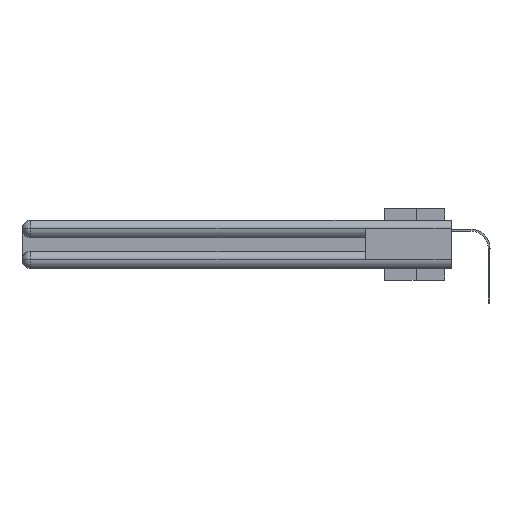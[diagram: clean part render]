
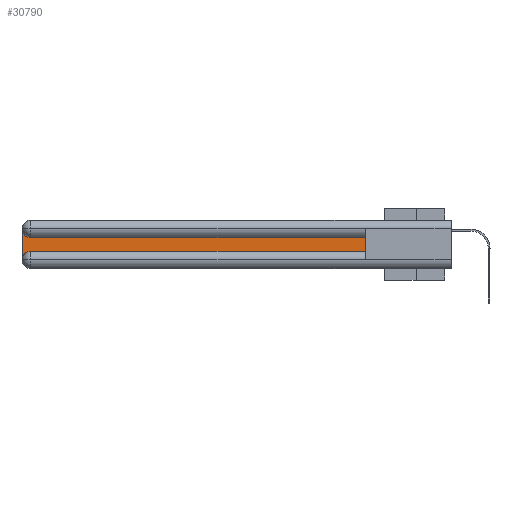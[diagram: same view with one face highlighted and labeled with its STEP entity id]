
A CAD part, left-side view. The second image highlights one B-rep face of the part: STEP entity #30790.
In plain terms, the highlighted planar face has unit normal (-1, 0, 0).
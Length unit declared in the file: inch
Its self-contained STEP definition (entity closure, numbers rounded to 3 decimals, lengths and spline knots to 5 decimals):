
#3 = EDGE_LOOP ( 'NONE', ( #7706, #17827, #25872, #24058, #19139, #547 ) ) ;
#547 = ORIENTED_EDGE ( 'NONE', *, *, #1718, .T. ) ;
#622 = DIRECTION ( 'NONE',  ( 0., 0., 1. ) ) ;
#997 = CARTESIAN_POINT ( 'NONE',  ( 0.075, 0.6, -0.1225 ) ) ;
#1361 = FACE_OUTER_BOUND ( 'NONE', #3, .T. ) ;
#1718 = EDGE_CURVE ( 'NONE', #11666, #32414, #20734, .T. ) ;
#3268 = VECTOR ( 'NONE', #26755, 39.37008 ) ;
#3394 = CARTESIAN_POINT ( 'NONE',  ( 0.075, 0.6, -0.1225 ) ) ;
#4124 = CARTESIAN_POINT ( 'NONE',  ( 0.075, 0.6, -0.2175 ) ) ;
#4169 = DIRECTION ( 'NONE',  ( 1., 0., 0. ) ) ;
#5726 = DIRECTION ( 'NONE',  ( 0., 0., -1. ) ) ;
#5893 = AXIS2_PLACEMENT_3D ( 'NONE', #29638, #4169, #29796 ) ;
#6067 = VERTEX_POINT ( 'NONE', #24082 ) ;
#6148 = VECTOR ( 'NONE', #622, 39.37008 ) ;
#6996 = PLANE ( 'NONE',  #32597 ) ;
#7706 = ORIENTED_EDGE ( 'NONE', *, *, #21511, .T. ) ;
#9807 = EDGE_CURVE ( 'NONE', #14120, #18936, #25700, .T. ) ;
#10392 = DIRECTION ( 'NONE',  ( 0., 0., -1. ) ) ;
#11161 = VECTOR ( 'NONE', #10392, 39.37008 ) ;
#11548 = CIRCLE ( 'NONE', #14212, 0.06 ) ;
#11666 = VERTEX_POINT ( 'NONE', #19000 ) ;
#12368 = EDGE_CURVE ( 'NONE', #18936, #6067, #11548, .T. ) ;
#13204 = CARTESIAN_POINT ( 'NONE',  ( 0.075, 3., -0.2175 ) ) ;
#13526 = CARTESIAN_POINT ( 'NONE',  ( 0.075, 3., -0.0625 ) ) ;
#13931 = VECTOR ( 'NONE', #23690, 39.37008 ) ;
#14120 = VERTEX_POINT ( 'NONE', #13526 ) ;
#14212 = AXIS2_PLACEMENT_3D ( 'NONE', #31208, #15884, #5726 ) ;
#15884 = DIRECTION ( 'NONE',  ( 1., 0., 0. ) ) ;
#17827 = ORIENTED_EDGE ( 'NONE', *, *, #20402, .T. ) ;
#18936 = VERTEX_POINT ( 'NONE', #27985 ) ;
#19000 = CARTESIAN_POINT ( 'NONE',  ( 0.075, 0.6, -0.2175 ) ) ;
#19139 = ORIENTED_EDGE ( 'NONE', *, *, #19537, .T. ) ;
#19537 = EDGE_CURVE ( 'NONE', #6067, #11666, #31924, .T. ) ;
#20239 = CIRCLE ( 'NONE', #5893, 0.06 ) ;
#20402 = EDGE_CURVE ( 'NONE', #32835, #14120, #20239, .T. ) ;
#20734 = LINE ( 'NONE', #23397, #6148 ) ;
#21511 = EDGE_CURVE ( 'NONE', #32414, #32835, #26023, .T. ) ;
#23397 = CARTESIAN_POINT ( 'NONE',  ( 0.075, 0.6, -0.2175 ) ) ;
#23690 = DIRECTION ( 'NONE',  ( 0., 1., 0. ) ) ;
#23736 = CARTESIAN_POINT ( 'NONE',  ( 0.075, 2.94, -0.1225 ) ) ;
#24058 = ORIENTED_EDGE ( 'NONE', *, *, #12368, .T. ) ;
#24082 = CARTESIAN_POINT ( 'NONE',  ( 0.075, 2.94, -0.2175 ) ) ;
#24305 = CARTESIAN_POINT ( 'NONE',  ( 0.075, 3., -0.1225 ) ) ;
#24640 = DIRECTION ( 'NONE',  ( 1., 0., 0. ) ) ;
#25700 = LINE ( 'NONE', #13204, #11161 ) ;
#25872 = ORIENTED_EDGE ( 'NONE', *, *, #9807, .T. ) ;
#26023 = LINE ( 'NONE', #3394, #13931 ) ;
#26755 = DIRECTION ( 'NONE',  ( 0., -1., 0. ) ) ;
#27985 = CARTESIAN_POINT ( 'NONE',  ( 0.075, 3., -0.2775 ) ) ;
#29638 = CARTESIAN_POINT ( 'NONE',  ( 0.075, 2.94, -0.0625 ) ) ;
#29796 = DIRECTION ( 'NONE',  ( 0., 0., -1. ) ) ;
#30790 = ADVANCED_FACE ( 'NONE', ( #1361 ), #6996, .F. ) ;
#31208 = CARTESIAN_POINT ( 'NONE',  ( 0.075, 2.94, -0.2775 ) ) ;
#31924 = LINE ( 'NONE', #4124, #3268 ) ;
#31984 = DIRECTION ( 'NONE',  ( 0., 0., -1. ) ) ;
#32414 = VERTEX_POINT ( 'NONE', #997 ) ;
#32597 = AXIS2_PLACEMENT_3D ( 'NONE', #24305, #24640, #31984 ) ;
#32835 = VERTEX_POINT ( 'NONE', #23736 ) ;
